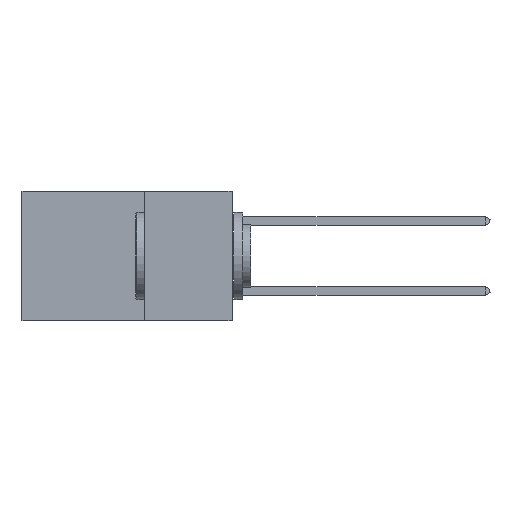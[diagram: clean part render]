
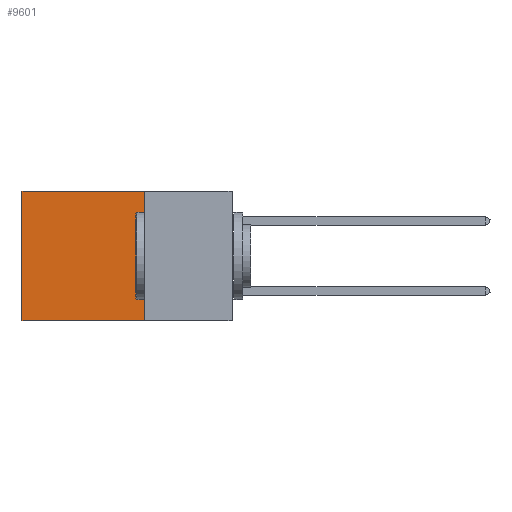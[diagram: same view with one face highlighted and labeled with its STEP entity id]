
A CAD part, left-side view. The second image highlights one B-rep face of the part: STEP entity #9601.
In plain terms, the highlighted planar face has unit normal (-1, 0, 0).
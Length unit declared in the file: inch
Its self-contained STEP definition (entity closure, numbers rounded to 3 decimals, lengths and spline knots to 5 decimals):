
#254 = AXIS2_PLACEMENT_3D ( 'NONE', #16234, #34241, #12750 ) ;
#1544 = ORIENTED_EDGE ( 'NONE', *, *, #25309, .F. ) ;
#2621 = EDGE_CURVE ( 'NONE', #24335, #28270, #20291, .T. ) ;
#3011 = DIRECTION ( 'NONE',  ( 0., 0., -1. ) ) ;
#5622 = ORIENTED_EDGE ( 'NONE', *, *, #2621, .T. ) ;
#9047 = PLANE ( 'NONE',  #254 ) ;
#9601 = ADVANCED_FACE ( 'NONE', ( #28256 ), #9047, .F. ) ;
#12393 = CARTESIAN_POINT ( 'NONE',  ( 0.2875, 0.6, 0. ) ) ;
#12750 = DIRECTION ( 'NONE',  ( 0., 0., -1. ) ) ;
#16234 = CARTESIAN_POINT ( 'NONE',  ( 0.2875, 0.25, 0. ) ) ;
#18267 = LINE ( 'NONE', #31950, #26673 ) ;
#20291 = LINE ( 'NONE', #43769, #38177 ) ;
#20718 = VECTOR ( 'NONE', #29726, 39.37008 ) ;
#20829 = VERTEX_POINT ( 'NONE', #41696 ) ;
#23838 = ORIENTED_EDGE ( 'NONE', *, *, #42968, .T. ) ;
#24335 = VERTEX_POINT ( 'NONE', #41759 ) ;
#25309 = EDGE_CURVE ( 'NONE', #24335, #44390, #18267, .T. ) ;
#26673 = VECTOR ( 'NONE', #3011, 39.37008 ) ;
#26790 = LINE ( 'NONE', #27910, #44671 ) ;
#27910 = CARTESIAN_POINT ( 'NONE',  ( 0.2875, 0.25, -0.37 ) ) ;
#28256 = FACE_OUTER_BOUND ( 'NONE', #32465, .T. ) ;
#28270 = VERTEX_POINT ( 'NONE', #12393 ) ;
#29139 = ORIENTED_EDGE ( 'NONE', *, *, #29817, .F. ) ;
#29726 = DIRECTION ( 'NONE',  ( 0., 0., -1. ) ) ;
#29817 = EDGE_CURVE ( 'NONE', #44390, #20829, #26790, .T. ) ;
#30253 = LINE ( 'NONE', #43929, #20718 ) ;
#31512 = DIRECTION ( 'NONE',  ( 0., 1., 0. ) ) ;
#31950 = CARTESIAN_POINT ( 'NONE',  ( 0.2875, 0.25, 0. ) ) ;
#32465 = EDGE_LOOP ( 'NONE', ( #23838, #29139, #1544, #5622 ) ) ;
#34241 = DIRECTION ( 'NONE',  ( 1., 0., 0. ) ) ;
#37059 = CARTESIAN_POINT ( 'NONE',  ( 0.2875, 0.25, -0.37 ) ) ;
#38177 = VECTOR ( 'NONE', #40189, 39.37008 ) ;
#40189 = DIRECTION ( 'NONE',  ( 0., 1., 0. ) ) ;
#41696 = CARTESIAN_POINT ( 'NONE',  ( 0.2875, 0.6, -0.37 ) ) ;
#41759 = CARTESIAN_POINT ( 'NONE',  ( 0.2875, 0.25, 0. ) ) ;
#42968 = EDGE_CURVE ( 'NONE', #28270, #20829, #30253, .T. ) ;
#43769 = CARTESIAN_POINT ( 'NONE',  ( 0.2875, 0.25, 0. ) ) ;
#43929 = CARTESIAN_POINT ( 'NONE',  ( 0.2875, 0.6, 0. ) ) ;
#44390 = VERTEX_POINT ( 'NONE', #37059 ) ;
#44671 = VECTOR ( 'NONE', #31512, 39.37008 ) ;
